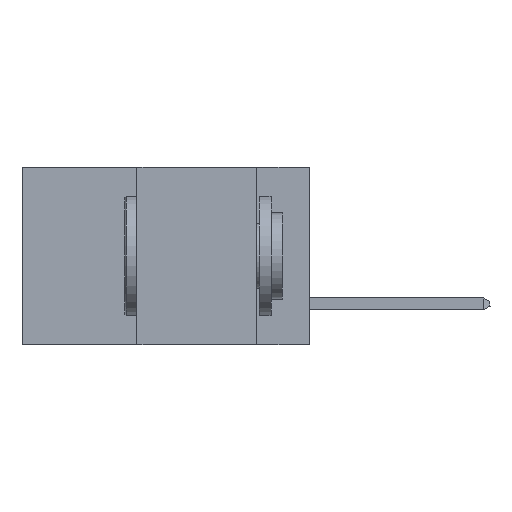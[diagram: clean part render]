
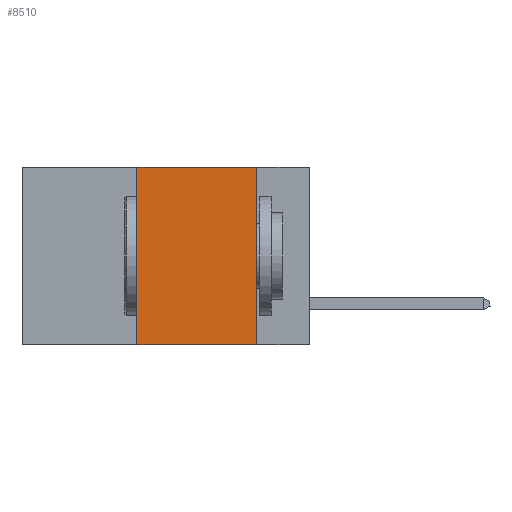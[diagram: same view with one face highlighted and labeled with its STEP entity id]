
A CAD part, left-side view. The second image highlights one B-rep face of the part: STEP entity #8510.
In plain terms, the highlighted planar face has unit normal (-1, 0, 0).
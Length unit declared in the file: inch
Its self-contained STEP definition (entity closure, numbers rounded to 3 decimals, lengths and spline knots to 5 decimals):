
#1689 = CARTESIAN_POINT ( 'NONE',  ( 0., 0.6, -0.37 ) ) ;
#2510 = CARTESIAN_POINT ( 'NONE',  ( 0., 0.6, 0. ) ) ;
#3290 = VERTEX_POINT ( 'NONE', #43538 ) ;
#3536 = CARTESIAN_POINT ( 'NONE',  ( 0., 0.36, 0. ) ) ;
#6828 = EDGE_CURVE ( 'NONE', #37977, #3290, #24334, .T. ) ;
#6831 = LINE ( 'NONE', #2510, #15846 ) ;
#7126 = LINE ( 'NONE', #29386, #36025 ) ;
#8510 = ADVANCED_FACE ( 'NONE', ( #36336 ), #10236, .F. ) ;
#9891 = DIRECTION ( 'NONE',  ( 0., -1., 0. ) ) ;
#10022 = VECTOR ( 'NONE', #30398, 39.37008 ) ;
#10074 = EDGE_CURVE ( 'NONE', #37977, #11422, #12446, .T. ) ;
#10236 = PLANE ( 'NONE',  #26722 ) ;
#11422 = VERTEX_POINT ( 'NONE', #34440 ) ;
#12446 = LINE ( 'NONE', #3536, #10022 ) ;
#13444 = ORIENTED_EDGE ( 'NONE', *, *, #10074, .F. ) ;
#14504 = EDGE_CURVE ( 'NONE', #36381, #3290, #7126, .T. ) ;
#15846 = VECTOR ( 'NONE', #9891, 39.37008 ) ;
#18318 = CARTESIAN_POINT ( 'NONE',  ( 0., 0.6, 0. ) ) ;
#24334 = LINE ( 'NONE', #1689, #30876 ) ;
#24504 = ORIENTED_EDGE ( 'NONE', *, *, #45402, .F. ) ;
#26720 = ORIENTED_EDGE ( 'NONE', *, *, #14504, .F. ) ;
#26722 = AXIS2_PLACEMENT_3D ( 'NONE', #18318, #29571, #45082 ) ;
#29386 = CARTESIAN_POINT ( 'NONE',  ( 0., 0.11, 0. ) ) ;
#29571 = DIRECTION ( 'NONE',  ( 1., 0., 0. ) ) ;
#30398 = DIRECTION ( 'NONE',  ( 0., 0., 1. ) ) ;
#30876 = VECTOR ( 'NONE', #39541, 39.37008 ) ;
#33038 = CARTESIAN_POINT ( 'NONE',  ( 0., 0.11, 0. ) ) ;
#34440 = CARTESIAN_POINT ( 'NONE',  ( 0., 0.36, 0. ) ) ;
#34717 = ORIENTED_EDGE ( 'NONE', *, *, #6828, .T. ) ;
#36025 = VECTOR ( 'NONE', #40690, 39.37008 ) ;
#36336 = FACE_OUTER_BOUND ( 'NONE', #37943, .T. ) ;
#36381 = VERTEX_POINT ( 'NONE', #33038 ) ;
#37943 = EDGE_LOOP ( 'NONE', ( #26720, #24504, #13444, #34717 ) ) ;
#37977 = VERTEX_POINT ( 'NONE', #43537 ) ;
#39541 = DIRECTION ( 'NONE',  ( 0., -1., 0. ) ) ;
#40690 = DIRECTION ( 'NONE',  ( 0., 0., -1. ) ) ;
#43537 = CARTESIAN_POINT ( 'NONE',  ( 0., 0.36, -0.37 ) ) ;
#43538 = CARTESIAN_POINT ( 'NONE',  ( 0., 0.11, -0.37 ) ) ;
#45082 = DIRECTION ( 'NONE',  ( 0., 0., -1. ) ) ;
#45402 = EDGE_CURVE ( 'NONE', #11422, #36381, #6831, .T. ) ;
